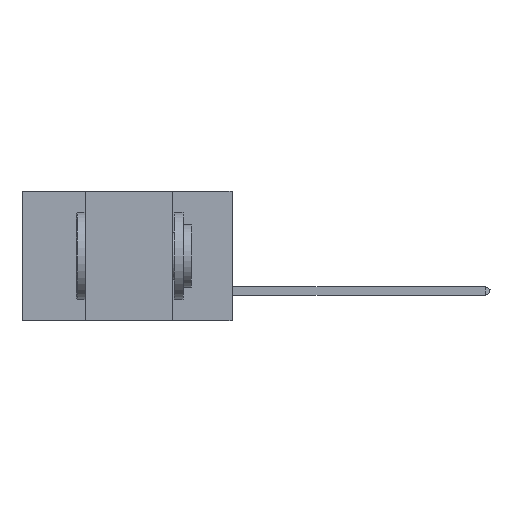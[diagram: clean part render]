
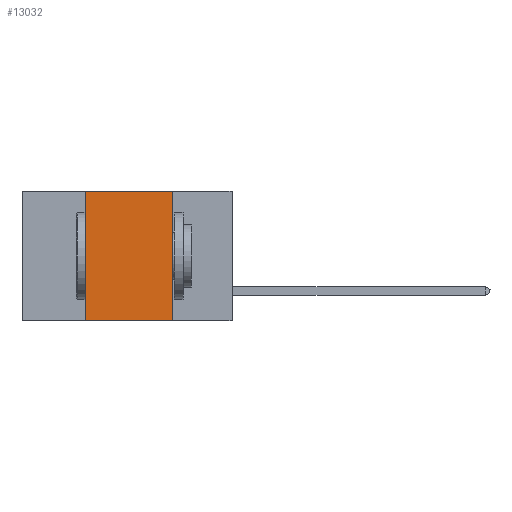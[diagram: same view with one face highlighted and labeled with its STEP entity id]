
A CAD part, left-side view. The second image highlights one B-rep face of the part: STEP entity #13032.
In plain terms, the highlighted planar face has unit normal (-1, 0, 0).
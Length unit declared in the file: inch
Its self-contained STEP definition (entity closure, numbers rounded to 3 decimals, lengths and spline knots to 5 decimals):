
#677 = ORIENTED_EDGE ( 'NONE', *, *, #28364, .F. ) ;
#4664 = AXIS2_PLACEMENT_3D ( 'NONE', #18848, #26833, #10980 ) ;
#4919 = VERTEX_POINT ( 'NONE', #23688 ) ;
#5216 = LINE ( 'NONE', #21312, #32505 ) ;
#7532 = VERTEX_POINT ( 'NONE', #33200 ) ;
#9050 = ORIENTED_EDGE ( 'NONE', *, *, #19925, .F. ) ;
#10524 = EDGE_CURVE ( 'NONE', #7532, #4919, #5216, .T. ) ;
#10980 = DIRECTION ( 'NONE',  ( 0., 0., -1. ) ) ;
#11333 = CARTESIAN_POINT ( 'NONE',  ( 0., 0.42, 0. ) ) ;
#12158 = CARTESIAN_POINT ( 'NONE',  ( 0., 0.6, -0.37 ) ) ;
#13032 = ADVANCED_FACE ( 'NONE', ( #16615 ), #13581, .F. ) ;
#13581 = PLANE ( 'NONE',  #4664 ) ;
#14276 = ORIENTED_EDGE ( 'NONE', *, *, #10524, .F. ) ;
#15126 = EDGE_CURVE ( 'NONE', #28992, #4919, #19670, .T. ) ;
#16615 = FACE_OUTER_BOUND ( 'NONE', #26961, .T. ) ;
#17061 = DIRECTION ( 'NONE',  ( 0., 0., 1. ) ) ;
#18848 = CARTESIAN_POINT ( 'NONE',  ( 0., 0.6, 0. ) ) ;
#19670 = LINE ( 'NONE', #12158, #23014 ) ;
#19925 = EDGE_CURVE ( 'NONE', #20513, #7532, #21034, .T. ) ;
#20513 = VERTEX_POINT ( 'NONE', #11333 ) ;
#20627 = VECTOR ( 'NONE', #20916, 39.37008 ) ;
#20916 = DIRECTION ( 'NONE',  ( 0., -1., 0. ) ) ;
#21034 = LINE ( 'NONE', #26339, #20627 ) ;
#21312 = CARTESIAN_POINT ( 'NONE',  ( 0., 0.17, 0. ) ) ;
#22032 = CARTESIAN_POINT ( 'NONE',  ( 0., 0.42, 0. ) ) ;
#23014 = VECTOR ( 'NONE', #30840, 39.37008 ) ;
#23688 = CARTESIAN_POINT ( 'NONE',  ( 0., 0.17, -0.37 ) ) ;
#24225 = ORIENTED_EDGE ( 'NONE', *, *, #15126, .T. ) ;
#26339 = CARTESIAN_POINT ( 'NONE',  ( 0., 0.6, 0. ) ) ;
#26833 = DIRECTION ( 'NONE',  ( 1., 0., 0. ) ) ;
#26961 = EDGE_LOOP ( 'NONE', ( #14276, #9050, #677, #24225 ) ) ;
#28364 = EDGE_CURVE ( 'NONE', #28992, #20513, #32608, .T. ) ;
#28992 = VERTEX_POINT ( 'NONE', #33014 ) ;
#29254 = DIRECTION ( 'NONE',  ( 0., 0., -1. ) ) ;
#30840 = DIRECTION ( 'NONE',  ( 0., -1., 0. ) ) ;
#32505 = VECTOR ( 'NONE', #29254, 39.37008 ) ;
#32608 = LINE ( 'NONE', #22032, #33004 ) ;
#33004 = VECTOR ( 'NONE', #17061, 39.37008 ) ;
#33014 = CARTESIAN_POINT ( 'NONE',  ( 0., 0.42, -0.37 ) ) ;
#33200 = CARTESIAN_POINT ( 'NONE',  ( 0., 0.17, 0. ) ) ;
